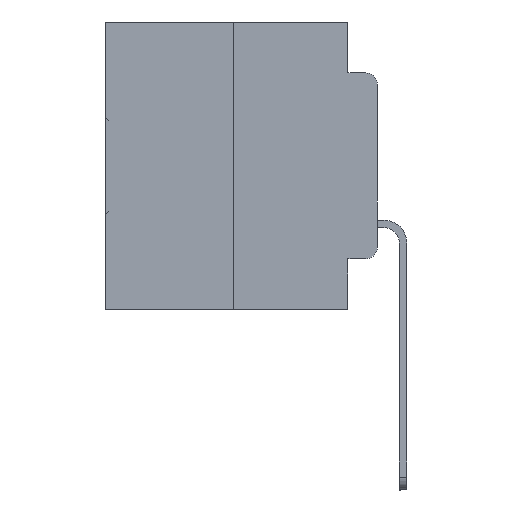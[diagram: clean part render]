
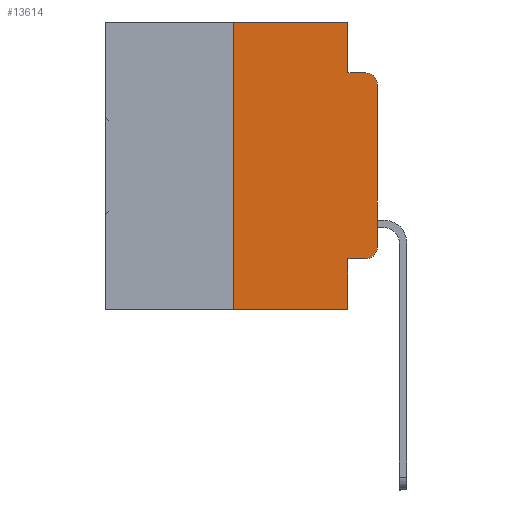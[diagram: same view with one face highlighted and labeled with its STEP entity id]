
A CAD part, left-side view. The second image highlights one B-rep face of the part: STEP entity #13614.
In plain terms, the highlighted planar face has unit normal (-1, 0, 0).
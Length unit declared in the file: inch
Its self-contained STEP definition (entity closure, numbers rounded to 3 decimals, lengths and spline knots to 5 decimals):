
#67 = CARTESIAN_POINT ( 'NONE',  ( 0., 0.02, -0.1085 ) ) ;
#522 = EDGE_CURVE ( 'NONE', #8508, #2183, #29417, .T. ) ;
#625 = CARTESIAN_POINT ( 'NONE',  ( 0., 0.473, -0.5 ) ) ;
#1222 = VECTOR ( 'NONE', #28859, 39.37008 ) ;
#1372 = CARTESIAN_POINT ( 'NONE',  ( 0., 0.051, -0.4115 ) ) ;
#1466 = ORIENTED_EDGE ( 'NONE', *, *, #24707, .T. ) ;
#1703 = CARTESIAN_POINT ( 'NONE',  ( 0., 0., -0.1085 ) ) ;
#2183 = VERTEX_POINT ( 'NONE', #3227 ) ;
#2672 = DIRECTION ( 'NONE',  ( 0., 0., -1. ) ) ;
#3227 = CARTESIAN_POINT ( 'NONE',  ( 0., 0.051, -0.5 ) ) ;
#3324 = CARTESIAN_POINT ( 'NONE',  ( 0., 0.051, -0.0885 ) ) ;
#3587 = CARTESIAN_POINT ( 'NONE',  ( 0., 0.051, -0.4115 ) ) ;
#3975 = EDGE_CURVE ( 'NONE', #5904, #10317, #30201, .T. ) ;
#3985 = LINE ( 'NONE', #3324, #16560 ) ;
#4273 = CARTESIAN_POINT ( 'NONE',  ( 0., 0.051, -0.0885 ) ) ;
#4513 = ORIENTED_EDGE ( 'NONE', *, *, #23514, .F. ) ;
#4557 = AXIS2_PLACEMENT_3D ( 'NONE', #12566, #29809, #15043 ) ;
#5052 = VERTEX_POINT ( 'NONE', #18932 ) ;
#5655 = LINE ( 'NONE', #10987, #24743 ) ;
#5741 = EDGE_CURVE ( 'NONE', #31335, #31071, #5655, .T. ) ;
#5904 = VERTEX_POINT ( 'NONE', #26549 ) ;
#5927 = DIRECTION ( 'NONE',  ( 0., -1., 0. ) ) ;
#7078 = EDGE_LOOP ( 'NONE', ( #23805, #26635, #25346, #21907, #4513, #18549, #31820, #27540, #1466, #7890 ) ) ;
#7263 = CARTESIAN_POINT ( 'NONE',  ( 0., 0.02, -0.0885 ) ) ;
#7475 = VECTOR ( 'NONE', #27456, 39.37008 ) ;
#7642 = CARTESIAN_POINT ( 'NONE',  ( 0., 0., 0. ) ) ;
#7744 = CARTESIAN_POINT ( 'NONE',  ( 0., 0.051, 0. ) ) ;
#7890 = ORIENTED_EDGE ( 'NONE', *, *, #14729, .T. ) ;
#8036 = LINE ( 'NONE', #1372, #1222 ) ;
#8129 = VECTOR ( 'NONE', #29569, 39.37008 ) ;
#8508 = VERTEX_POINT ( 'NONE', #3587 ) ;
#8940 = LINE ( 'NONE', #16546, #25593 ) ;
#9111 = CARTESIAN_POINT ( 'NONE',  ( 0., 0.051, 0. ) ) ;
#9130 = EDGE_CURVE ( 'NONE', #31071, #15321, #3985, .T. ) ;
#10317 = VERTEX_POINT ( 'NONE', #13631 ) ;
#10515 = VECTOR ( 'NONE', #21585, 39.37008 ) ;
#10860 = CIRCLE ( 'NONE', #11150, 0.02 ) ;
#10987 = CARTESIAN_POINT ( 'NONE',  ( 0., 0.051, 0. ) ) ;
#11150 = AXIS2_PLACEMENT_3D ( 'NONE', #27329, #12534, #29782 ) ;
#11394 = CARTESIAN_POINT ( 'NONE',  ( 0., 0., -0.3915 ) ) ;
#12464 = EDGE_CURVE ( 'NONE', #21337, #15321, #21434, .T. ) ;
#12534 = DIRECTION ( 'NONE',  ( -1., 0., 0. ) ) ;
#12566 = CARTESIAN_POINT ( 'NONE',  ( 0., 0.473, 0. ) ) ;
#13614 = ADVANCED_FACE ( 'NONE', ( #14348 ), #27362, .F. ) ;
#13631 = CARTESIAN_POINT ( 'NONE',  ( 0., 0.25, 0. ) ) ;
#14348 = FACE_OUTER_BOUND ( 'NONE', #7078, .T. ) ;
#14729 = EDGE_CURVE ( 'NONE', #5052, #27765, #10860, .T. ) ;
#14953 = EDGE_CURVE ( 'NONE', #5904, #2183, #23652, .T. ) ;
#15043 = DIRECTION ( 'NONE',  ( 0., 0., -1. ) ) ;
#15321 = VERTEX_POINT ( 'NONE', #7263 ) ;
#16546 = CARTESIAN_POINT ( 'NONE',  ( 0., 0.473, 0. ) ) ;
#16560 = VECTOR ( 'NONE', #5927, 39.37008 ) ;
#17744 = DIRECTION ( 'NONE',  ( -1., 0., 0. ) ) ;
#18549 = ORIENTED_EDGE ( 'NONE', *, *, #3975, .F. ) ;
#18932 = CARTESIAN_POINT ( 'NONE',  ( 0., 0.02, -0.4115 ) ) ;
#19062 = DIRECTION ( 'NONE',  ( 0., -1., 0. ) ) ;
#19103 = CARTESIAN_POINT ( 'NONE',  ( 0., 0.25, 0. ) ) ;
#19114 = EDGE_CURVE ( 'NONE', #27765, #21337, #21486, .T. ) ;
#21337 = VERTEX_POINT ( 'NONE', #1703 ) ;
#21434 = CIRCLE ( 'NONE', #26031, 0.02 ) ;
#21486 = LINE ( 'NONE', #7642, #7475 ) ;
#21585 = DIRECTION ( 'NONE',  ( 0., 0., 1. ) ) ;
#21907 = ORIENTED_EDGE ( 'NONE', *, *, #5741, .F. ) ;
#23514 = EDGE_CURVE ( 'NONE', #10317, #31335, #8940, .T. ) ;
#23652 = LINE ( 'NONE', #625, #30143 ) ;
#23805 = ORIENTED_EDGE ( 'NONE', *, *, #19114, .T. ) ;
#24707 = EDGE_CURVE ( 'NONE', #8508, #5052, #8036, .T. ) ;
#24743 = VECTOR ( 'NONE', #28278, 39.37008 ) ;
#25346 = ORIENTED_EDGE ( 'NONE', *, *, #9130, .F. ) ;
#25593 = VECTOR ( 'NONE', #19062, 39.37008 ) ;
#25717 = DIRECTION ( 'NONE',  ( 0., -1., 0. ) ) ;
#26031 = AXIS2_PLACEMENT_3D ( 'NONE', #67, #17744, #2672 ) ;
#26549 = CARTESIAN_POINT ( 'NONE',  ( 0., 0.25, -0.5 ) ) ;
#26635 = ORIENTED_EDGE ( 'NONE', *, *, #12464, .T. ) ;
#27329 = CARTESIAN_POINT ( 'NONE',  ( 0., 0.02, -0.3915 ) ) ;
#27362 = PLANE ( 'NONE',  #4557 ) ;
#27456 = DIRECTION ( 'NONE',  ( 0., 0., 1. ) ) ;
#27540 = ORIENTED_EDGE ( 'NONE', *, *, #522, .F. ) ;
#27765 = VERTEX_POINT ( 'NONE', #11394 ) ;
#28278 = DIRECTION ( 'NONE',  ( 0., 0., -1. ) ) ;
#28859 = DIRECTION ( 'NONE',  ( 0., -1., 0. ) ) ;
#29417 = LINE ( 'NONE', #9111, #8129 ) ;
#29569 = DIRECTION ( 'NONE',  ( 0., 0., -1. ) ) ;
#29782 = DIRECTION ( 'NONE',  ( 0., 0., -1. ) ) ;
#29809 = DIRECTION ( 'NONE',  ( 1., 0., 0. ) ) ;
#30143 = VECTOR ( 'NONE', #25717, 39.37008 ) ;
#30201 = LINE ( 'NONE', #19103, #10515 ) ;
#31071 = VERTEX_POINT ( 'NONE', #4273 ) ;
#31335 = VERTEX_POINT ( 'NONE', #7744 ) ;
#31820 = ORIENTED_EDGE ( 'NONE', *, *, #14953, .T. ) ;
